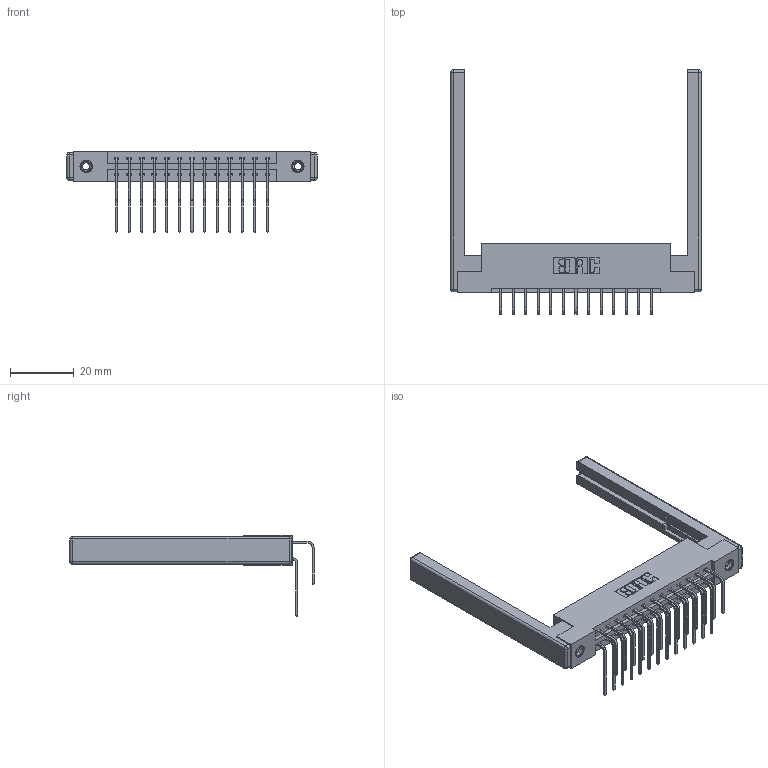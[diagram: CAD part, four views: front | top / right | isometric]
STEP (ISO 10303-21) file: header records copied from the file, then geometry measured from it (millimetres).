
FILE_DESCRIPTION (( 'STEP AP203' ), '1' );
FILE_NAME ('387-026-558-268.STEP', '2019-10-16T20:53:04', ( '' ), ( '' ), 'SwSTEP 2.0', 'SolidWorks 2016', '' );
FILE_SCHEMA (( 'CONFIG_CONTROL_DESIGN' ));
Length unit declared in the file: inch
Products named in the file (6): 337 Part_Flush Mounting Lugs - 0.156 Dia-TI; 345-250-001_345-250-001-102; 345-292-001_558 Tail - 2; 387-026-558-268; 345-292-001_558 559 Tail - 1; 307-220-068
Assembly tree (31 placements, depth 2):
  387-026-558-268
    337 Part_Flush Mounting Lugs - 0.156 Dia-TI
    345-292-001_558 559 Tail - 1  x13
    345-292-001_558 Tail - 2  x13
    345-250-001_345-250-001-102  x2
    307-220-068  x2
Bounding box: 78.94 x 76.9 x 25.53 mm (x, y, z)
Volume: 12468.4 mm3; surface area: 13644.3 mm2
Topology: 31 solids, 31 shells, 1724 faces, 5043 edges, 3306 vertices
Faces by surface type: plane 1198, cylinder 502, cone 12, sphere 8, torus 4
Entity records: 18374 total; most frequent: CARTESIAN_POINT 3130, ORIENTED_EDGE 3004, DIRECTION 2768, EDGE_CURVE 1502, VECTOR 1284, LINE 1284, VERTEX_POINT 990, AXIS2_PLACEMENT_3D 742
